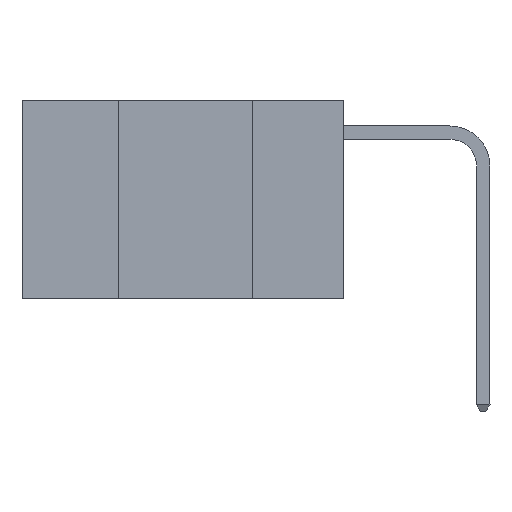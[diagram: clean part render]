
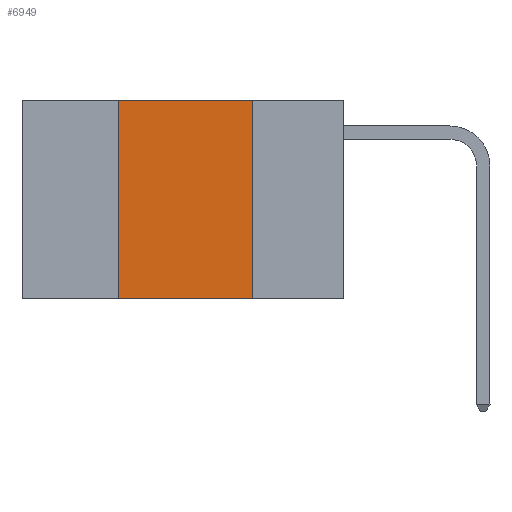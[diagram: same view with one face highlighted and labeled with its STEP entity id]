
A CAD part, left-side view. The second image highlights one B-rep face of the part: STEP entity #6949.
In plain terms, the highlighted planar face has unit normal (-1, 0, 0).
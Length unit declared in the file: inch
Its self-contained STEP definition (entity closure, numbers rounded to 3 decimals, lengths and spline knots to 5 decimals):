
#143 = VECTOR ( 'NONE', #281, 39.37008 ) ;
#281 = DIRECTION ( 'NONE',  ( 0., 0., 1. ) ) ;
#299 = DIRECTION ( 'NONE',  ( 0., -1., 0. ) ) ;
#338 = LINE ( 'NONE', #8988, #6660 ) ;
#363 = LINE ( 'NONE', #15084, #143 ) ;
#703 = VERTEX_POINT ( 'NONE', #5933 ) ;
#899 = CARTESIAN_POINT ( 'NONE',  ( 0., 0.17, 0. ) ) ;
#1196 = ORIENTED_EDGE ( 'NONE', *, *, #8930, .T. ) ;
#2209 = VERTEX_POINT ( 'NONE', #15328 ) ;
#2344 = PLANE ( 'NONE',  #12820 ) ;
#3242 = CARTESIAN_POINT ( 'NONE',  ( 0., 0.42, -0.37 ) ) ;
#3933 = LINE ( 'NONE', #8869, #6703 ) ;
#4223 = LINE ( 'NONE', #9006, #7973 ) ;
#5933 = CARTESIAN_POINT ( 'NONE',  ( 0., 0.42, 0. ) ) ;
#6228 = EDGE_CURVE ( 'NONE', #10733, #703, #363, .T. ) ;
#6375 = ORIENTED_EDGE ( 'NONE', *, *, #11558, .F. ) ;
#6660 = VECTOR ( 'NONE', #12642, 39.37008 ) ;
#6703 = VECTOR ( 'NONE', #299, 39.37008 ) ;
#6949 = ADVANCED_FACE ( 'NONE', ( #10835 ), #2344, .F. ) ;
#7614 = DIRECTION ( 'NONE',  ( 1., 0., 0. ) ) ;
#7803 = ORIENTED_EDGE ( 'NONE', *, *, #9323, .F. ) ;
#7973 = VECTOR ( 'NONE', #11680, 39.37008 ) ;
#8646 = CARTESIAN_POINT ( 'NONE',  ( 0., 0.6, 0. ) ) ;
#8869 = CARTESIAN_POINT ( 'NONE',  ( 0., 0.6, 0. ) ) ;
#8930 = EDGE_CURVE ( 'NONE', #10733, #2209, #4223, .T. ) ;
#8988 = CARTESIAN_POINT ( 'NONE',  ( 0., 0.17, 0. ) ) ;
#9006 = CARTESIAN_POINT ( 'NONE',  ( 0., 0.6, -0.37 ) ) ;
#9323 = EDGE_CURVE ( 'NONE', #15902, #2209, #338, .T. ) ;
#9951 = DIRECTION ( 'NONE',  ( 0., 0., -1. ) ) ;
#10733 = VERTEX_POINT ( 'NONE', #3242 ) ;
#10835 = FACE_OUTER_BOUND ( 'NONE', #13627, .T. ) ;
#11493 = ORIENTED_EDGE ( 'NONE', *, *, #6228, .F. ) ;
#11558 = EDGE_CURVE ( 'NONE', #703, #15902, #3933, .T. ) ;
#11680 = DIRECTION ( 'NONE',  ( 0., -1., 0. ) ) ;
#12642 = DIRECTION ( 'NONE',  ( 0., 0., -1. ) ) ;
#12820 = AXIS2_PLACEMENT_3D ( 'NONE', #8646, #7614, #9951 ) ;
#13627 = EDGE_LOOP ( 'NONE', ( #7803, #6375, #11493, #1196 ) ) ;
#15084 = CARTESIAN_POINT ( 'NONE',  ( 0., 0.42, 0. ) ) ;
#15328 = CARTESIAN_POINT ( 'NONE',  ( 0., 0.17, -0.37 ) ) ;
#15902 = VERTEX_POINT ( 'NONE', #899 ) ;
